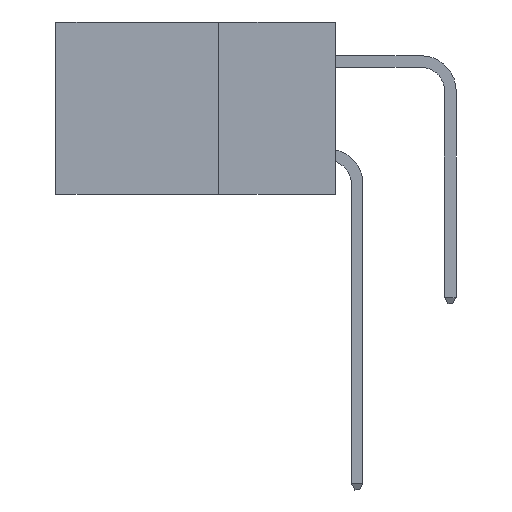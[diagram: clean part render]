
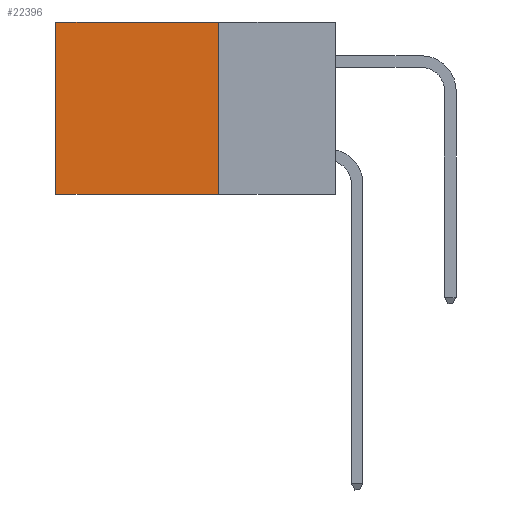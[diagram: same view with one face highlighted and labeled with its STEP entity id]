
A CAD part, left-side view. The second image highlights one B-rep face of the part: STEP entity #22396.
In plain terms, the highlighted planar face has unit normal (-1, 0, 0).
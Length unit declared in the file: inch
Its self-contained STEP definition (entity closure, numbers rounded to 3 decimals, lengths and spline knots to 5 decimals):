
#35 = LINE ( 'NONE', #7595, #17859 ) ;
#444 = EDGE_CURVE ( 'NONE', #8415, #18856, #11144, .T. ) ;
#807 = FACE_OUTER_BOUND ( 'NONE', #14829, .T. ) ;
#1098 = VERTEX_POINT ( 'NONE', #1841 ) ;
#1290 = EDGE_CURVE ( 'NONE', #1098, #19914, #35, .T. ) ;
#1841 = CARTESIAN_POINT ( 'NONE',  ( 0.2875, 0.6, 0. ) ) ;
#2028 = CARTESIAN_POINT ( 'NONE',  ( 0.2875, 0.25, -0.37 ) ) ;
#2865 = EDGE_CURVE ( 'NONE', #8415, #1098, #16090, .T. ) ;
#2891 = ORIENTED_EDGE ( 'NONE', *, *, #2865, .T. ) ;
#4070 = VECTOR ( 'NONE', #10978, 39.37008 ) ;
#4092 = DIRECTION ( 'NONE',  ( 0., 1., 0. ) ) ;
#4155 = EDGE_CURVE ( 'NONE', #18856, #19914, #10725, .T. ) ;
#5863 = DIRECTION ( 'NONE',  ( 0., 0., -1. ) ) ;
#5916 = VECTOR ( 'NONE', #12779, 39.37008 ) ;
#5976 = ORIENTED_EDGE ( 'NONE', *, *, #4155, .F. ) ;
#7595 = CARTESIAN_POINT ( 'NONE',  ( 0.2875, 0.6, 0. ) ) ;
#7878 = VECTOR ( 'NONE', #4092, 39.37008 ) ;
#8415 = VERTEX_POINT ( 'NONE', #15360 ) ;
#9626 = CARTESIAN_POINT ( 'NONE',  ( 0.2875, 0.25, 0. ) ) ;
#10725 = LINE ( 'NONE', #21549, #5916 ) ;
#10978 = DIRECTION ( 'NONE',  ( 0., 0., -1. ) ) ;
#11144 = LINE ( 'NONE', #23104, #4070 ) ;
#12779 = DIRECTION ( 'NONE',  ( 0., 1., 0. ) ) ;
#13734 = CARTESIAN_POINT ( 'NONE',  ( 0.2875, 0.6, -0.37 ) ) ;
#13929 = CARTESIAN_POINT ( 'NONE',  ( 0.2875, 0.25, 0. ) ) ;
#14652 = AXIS2_PLACEMENT_3D ( 'NONE', #13929, #23003, #22933 ) ;
#14829 = EDGE_LOOP ( 'NONE', ( #21196, #5976, #15183, #2891 ) ) ;
#15183 = ORIENTED_EDGE ( 'NONE', *, *, #444, .F. ) ;
#15360 = CARTESIAN_POINT ( 'NONE',  ( 0.2875, 0.25, 0. ) ) ;
#16090 = LINE ( 'NONE', #9626, #7878 ) ;
#17406 = PLANE ( 'NONE',  #14652 ) ;
#17859 = VECTOR ( 'NONE', #5863, 39.37008 ) ;
#18856 = VERTEX_POINT ( 'NONE', #2028 ) ;
#19914 = VERTEX_POINT ( 'NONE', #13734 ) ;
#21196 = ORIENTED_EDGE ( 'NONE', *, *, #1290, .T. ) ;
#21549 = CARTESIAN_POINT ( 'NONE',  ( 0.2875, 0.25, -0.37 ) ) ;
#22396 = ADVANCED_FACE ( 'NONE', ( #807 ), #17406, .F. ) ;
#22933 = DIRECTION ( 'NONE',  ( 0., 0., -1. ) ) ;
#23003 = DIRECTION ( 'NONE',  ( 1., 0., 0. ) ) ;
#23104 = CARTESIAN_POINT ( 'NONE',  ( 0.2875, 0.25, 0. ) ) ;
